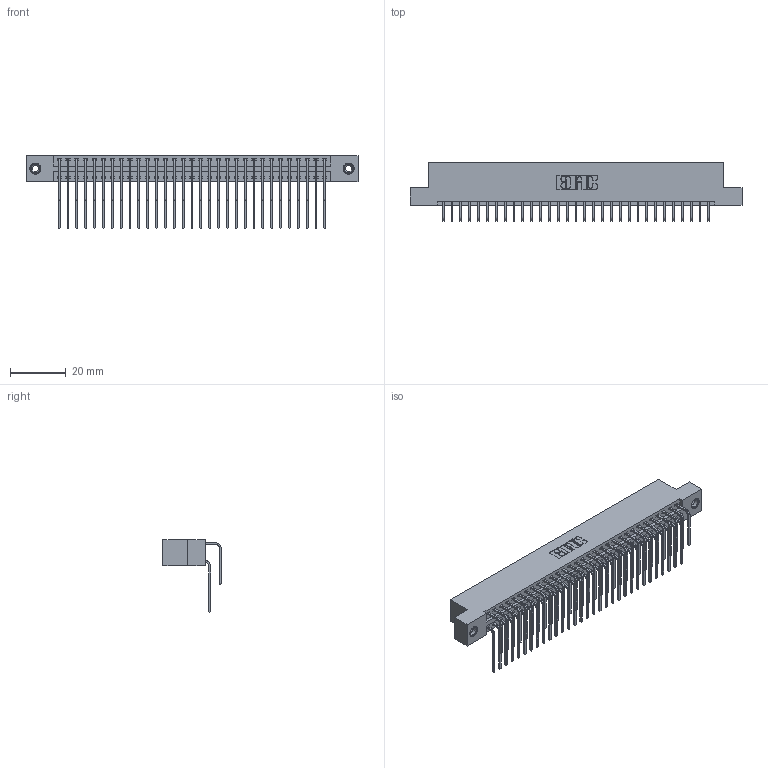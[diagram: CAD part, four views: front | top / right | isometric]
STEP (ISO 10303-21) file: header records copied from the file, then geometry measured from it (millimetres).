
FILE_DESCRIPTION (( 'STEP AP203' ), '1' );
FILE_NAME ('346-062-559-208.STEP', '2022-05-24T14:27:17', ( '' ), ( '' ), 'SwSTEP 2.0', 'SolidWorks 2020', '' );
FILE_SCHEMA (( 'CONFIG_CONTROL_DESIGN' ));
Length unit declared in the file: inch
Products named in the file (5): 345-292-001_558 559 Tail - 1; 345-250-001_345-250-003-102; 345-292-001_559 Tail - 2; 346-062-559-208; 346 Part_Flush Mounting Lugs - 0.156 Dia-TI
Assembly tree (65 placements, depth 2):
  346-062-559-208
    346 Part_Flush Mounting Lugs - 0.156 Dia-TI
    345-292-001_558 559 Tail - 1  x31
    345-292-001_559 Tail - 2  x31
    345-250-001_345-250-003-102  x2
Bounding box: 119 x 20.89 x 26.16 mm (x, y, z)
Volume: 11869.6 mm3; surface area: 17878.5 mm2
Topology: 65 solids, 65 shells, 3530 faces, 10447 edges, 6874 vertices
Faces by surface type: plane 2402, cylinder 1112, cone 12, torus 4
Entity records: 24682 total; most frequent: CARTESIAN_POINT 4118, ORIENTED_EDGE 3994, DIRECTION 3679, EDGE_CURVE 1997, LINE 1681, VECTOR 1681, VERTEX_POINT 1324, AXIS2_PLACEMENT_3D 999
